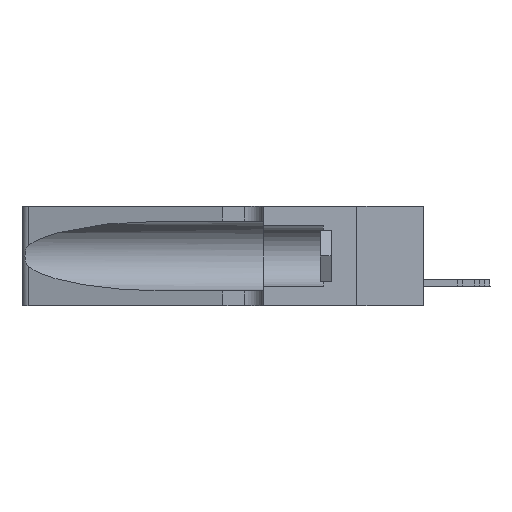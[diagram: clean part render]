
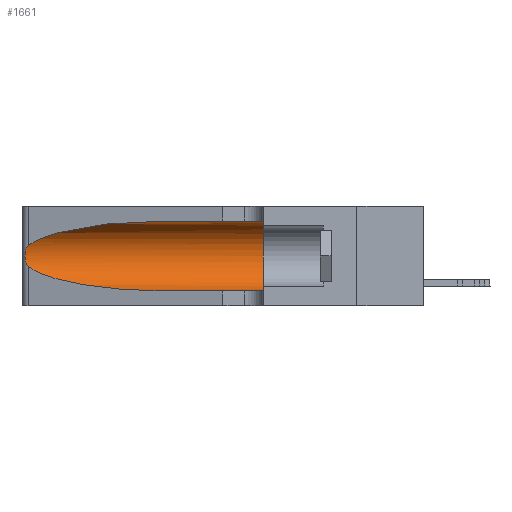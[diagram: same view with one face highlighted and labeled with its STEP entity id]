
A CAD part, left-side view. The second image highlights one B-rep face of the part: STEP entity #1661.
In plain terms, the highlighted cylindrical face has radius 3.308 mm (diameter 6.617 mm), a partial arc.
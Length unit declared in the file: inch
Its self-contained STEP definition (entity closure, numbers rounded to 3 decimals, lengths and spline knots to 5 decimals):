
#984 = ORIENTED_EDGE ( 'NONE', *, *, #26112, .T. ) ;
#1270 = AXIS2_PLACEMENT_3D ( 'NONE', #8919, #40380, #16643 ) ;
#1661 = ADVANCED_FACE ( 'NONE', ( #10866 ), #5829, .F. ) ;
#3133 = CARTESIAN_POINT ( 'NONE',  ( 0.25487, 1.22718, 0.22369 ) ) ;
#3387 = ORIENTED_EDGE ( 'NONE', *, *, #31826, .F. ) ;
#4576 = ORIENTED_EDGE ( 'NONE', *, *, #33304, .T. ) ;
#5829 = CYLINDRICAL_SURFACE ( 'NONE', #1270, 0.13025 ) ;
#7027 = CARTESIAN_POINT ( 'NONE',  ( 0.25487, 1.22718, 0.14631 ) ) ;
#7042 = ORIENTED_EDGE ( 'NONE', *, *, #17360, .T. ) ;
#7273 = CARTESIAN_POINT ( 'NONE',  ( 0.2373, 1.15595, 0.28018 ) ) ;
#8141 = CARTESIAN_POINT ( 'NONE',  ( 0.18966, 0.96281, 0.05475 ) ) ;
#8919 = CARTESIAN_POINT ( 'NONE',  ( 0.1305, 1.61858, 0.185 ) ) ;
#8937 = AXIS2_PLACEMENT_3D ( 'NONE', #37405, #23372, #17646 ) ;
#10866 = FACE_OUTER_BOUND ( 'NONE', #15667, .T. ) ;
#11171 = CARTESIAN_POINT ( 'NONE',  ( 0.25854, 1.2359, 0.20912 ) ) ;
#11788 = VERTEX_POINT ( 'NONE', #24856 ) ;
#14259 = ORIENTED_EDGE ( 'NONE', *, *, #26682, .T. ) ;
#14264 = EDGE_CURVE ( 'NONE', #21115, #38032, #42247, .T. ) ;
#14957 = CARTESIAN_POINT ( 'NONE',  ( 0.2373, 1.15595, 0.08982 ) ) ;
#15429 = CARTESIAN_POINT ( 'NONE',  ( 0.1305, 0.72297, 0.05475 ) ) ;
#15667 = EDGE_LOOP ( 'NONE', ( #7042, #4576, #984, #14259, #28988, #3387 ) ) ;
#16643 = DIRECTION ( 'NONE',  ( 0., 0., -1. ) ) ;
#17360 = EDGE_CURVE ( 'NONE', #20398, #24964, #32159, .T. ) ;
#17646 = DIRECTION ( 'NONE',  ( 0., 0., 1. ) ) ;
#18797 = CARTESIAN_POINT ( 'NONE',  ( 0.18966, 0.96281, 0.31525 ) ) ;
#18808 = DIRECTION ( 'NONE',  ( 0., -1., 0. ) ) ;
#19099 = CARTESIAN_POINT ( 'NONE',  ( 0.1305, 0.35, 0.31525 ) ) ;
#20319 = CARTESIAN_POINT ( 'NONE',  ( 0.25487, 1.22718, 0.22369 ) ) ;
#20398 = VERTEX_POINT ( 'NONE', #21040 ) ;
#21040 = CARTESIAN_POINT ( 'NONE',  ( 0.1305, 0.72297, 0.31525 ) ) ;
#21115 = VERTEX_POINT ( 'NONE', #19099 ) ;
#23372 = DIRECTION ( 'NONE',  ( 0., 1., 0. ) ) ;
#23705 =( BOUNDED_CURVE ( )  B_SPLINE_CURVE ( 3, ( #7027, #14957, #8141, #15429 ),
 .UNSPECIFIED., .F., .F. ) 
 B_SPLINE_CURVE_WITH_KNOTS ( ( 4, 4 ),
 ( 3.44316, 4.71239 ),
 .UNSPECIFIED. ) 
 CURVE ( )  GEOMETRIC_REPRESENTATION_ITEM ( )  RATIONAL_B_SPLINE_CURVE ( ( 1., 0.87, 0.87, 1. ) ) 
 REPRESENTATION_ITEM ( '' )  );
#24211 = LINE ( 'NONE', #50512, #45814 ) ;
#24213 = B_SPLINE_CURVE_WITH_KNOTS ( 'NONE', 3,
 ( #20319, #49194, #47937, #39489, #11171, #48486, #27441, #50776, #48570, #36852, #43656, #28034, #32327, #28205 ),
 .UNSPECIFIED., .F., .F.,
 ( 4, 2, 2, 2, 2, 2, 4 ),
 ( 0., 0.00027, 0.00053, 0.00107, 0.0016, 0.00187, 0.00214 ),
 .UNSPECIFIED. ) ;
#24856 = CARTESIAN_POINT ( 'NONE',  ( 0.1305, 0.72297, 0.05475 ) ) ;
#24964 = VERTEX_POINT ( 'NONE', #44459 ) ;
#26112 = EDGE_CURVE ( 'NONE', #46206, #11788, #23705, .T. ) ;
#26682 = EDGE_CURVE ( 'NONE', #11788, #38032, #24211, .T. ) ;
#27396 = CARTESIAN_POINT ( 'NONE',  ( 0.1305, 0.72297, 0.31525 ) ) ;
#27441 = CARTESIAN_POINT ( 'NONE',  ( 0.26075, 1.23896, 0.19203 ) ) ;
#28034 = CARTESIAN_POINT ( 'NONE',  ( 0.25639, 1.23186, 0.15144 ) ) ;
#28205 = CARTESIAN_POINT ( 'NONE',  ( 0.25487, 1.22718, 0.14631 ) ) ;
#28988 = ORIENTED_EDGE ( 'NONE', *, *, #14264, .F. ) ;
#29781 = DIRECTION ( 'NONE',  ( 0., -1., 0. ) ) ;
#31826 = EDGE_CURVE ( 'NONE', #20398, #21115, #36323, .T. ) ;
#32159 =( BOUNDED_CURVE ( )  B_SPLINE_CURVE ( 3, ( #27396, #18797, #7273, #3133 ),
 .UNSPECIFIED., .F., .T. ) 
 B_SPLINE_CURVE_WITH_KNOTS ( ( 4, 4 ),
 ( 1.5708, 2.84003 ),
 .UNSPECIFIED. ) 
 CURVE ( )  GEOMETRIC_REPRESENTATION_ITEM ( )  RATIONAL_B_SPLINE_CURVE ( ( 1., 0.87, 0.87, 1. ) ) 
 REPRESENTATION_ITEM ( '' )  );
#32327 = CARTESIAN_POINT ( 'NONE',  ( 0.25555, 1.22993, 0.14849 ) ) ;
#33304 = EDGE_CURVE ( 'NONE', #24964, #46206, #24213, .T. ) ;
#34121 = CARTESIAN_POINT ( 'NONE',  ( 0.1305, 0.35, 0.05475 ) ) ;
#35199 = VECTOR ( 'NONE', #29781, 39.37008 ) ;
#36323 = LINE ( 'NONE', #49196, #35199 ) ;
#36852 = CARTESIAN_POINT ( 'NONE',  ( 0.25856, 1.23593, 0.16098 ) ) ;
#37405 = CARTESIAN_POINT ( 'NONE',  ( 0.1305, 0.35, 0.185 ) ) ;
#38032 = VERTEX_POINT ( 'NONE', #34121 ) ;
#39489 = CARTESIAN_POINT ( 'NONE',  ( 0.25787, 1.23484, 0.2124 ) ) ;
#39532 = CARTESIAN_POINT ( 'NONE',  ( 0.25487, 1.22718, 0.14631 ) ) ;
#40380 = DIRECTION ( 'NONE',  ( 0., -1., 0. ) ) ;
#42247 = CIRCLE ( 'NONE', #8937, 0.13025 ) ;
#43656 = CARTESIAN_POINT ( 'NONE',  ( 0.25789, 1.23486, 0.15765 ) ) ;
#44459 = CARTESIAN_POINT ( 'NONE',  ( 0.25487, 1.22718, 0.22369 ) ) ;
#45814 = VECTOR ( 'NONE', #18808, 39.37008 ) ;
#46206 = VERTEX_POINT ( 'NONE', #39532 ) ;
#47937 = CARTESIAN_POINT ( 'NONE',  ( 0.25639, 1.23184, 0.21858 ) ) ;
#48486 = CARTESIAN_POINT ( 'NONE',  ( 0.26018, 1.23835, 0.19895 ) ) ;
#48570 = CARTESIAN_POINT ( 'NONE',  ( 0.26017, 1.23833, 0.17102 ) ) ;
#49194 = CARTESIAN_POINT ( 'NONE',  ( 0.25555, 1.22994, 0.2215 ) ) ;
#49196 = CARTESIAN_POINT ( 'NONE',  ( 0.1305, 1.61858, 0.31525 ) ) ;
#50512 = CARTESIAN_POINT ( 'NONE',  ( 0.1305, 1.61858, 0.05475 ) ) ;
#50776 = CARTESIAN_POINT ( 'NONE',  ( 0.26075, 1.23896, 0.178 ) ) ;
